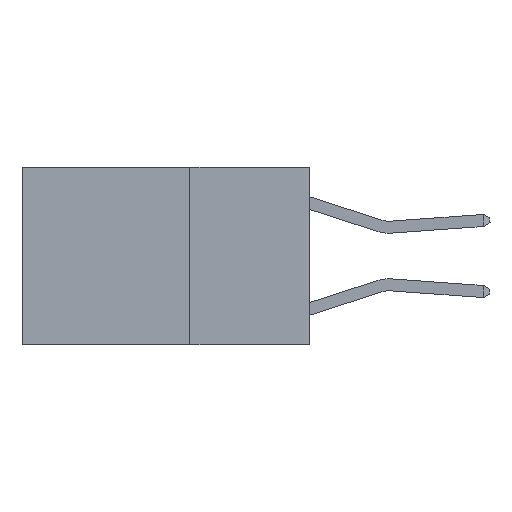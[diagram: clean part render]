
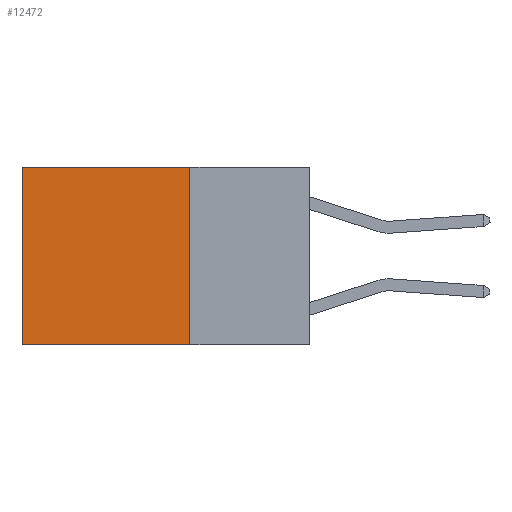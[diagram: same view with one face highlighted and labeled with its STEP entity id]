
A CAD part, left-side view. The second image highlights one B-rep face of the part: STEP entity #12472.
In plain terms, the highlighted planar face has unit normal (-1, 0, 0).
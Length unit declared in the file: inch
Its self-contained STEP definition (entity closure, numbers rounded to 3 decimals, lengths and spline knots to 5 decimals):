
#630 = CARTESIAN_POINT ( 'NONE',  ( 0.2625, 0.25, 0. ) ) ;
#1716 = LINE ( 'NONE', #6761, #12873 ) ;
#1860 = VECTOR ( 'NONE', #16292, 39.37008 ) ;
#2094 = VERTEX_POINT ( 'NONE', #2474 ) ;
#2474 = CARTESIAN_POINT ( 'NONE',  ( 0.2625, 0.6, -0.37 ) ) ;
#2919 = FACE_OUTER_BOUND ( 'NONE', #8704, .T. ) ;
#2928 = LINE ( 'NONE', #9169, #17981 ) ;
#3187 = CARTESIAN_POINT ( 'NONE',  ( 0.2625, 0.25, 0. ) ) ;
#3394 = ORIENTED_EDGE ( 'NONE', *, *, #8273, .F. ) ;
#3445 = CARTESIAN_POINT ( 'NONE',  ( 0.2625, 0.25, -0.37 ) ) ;
#4412 = VERTEX_POINT ( 'NONE', #630 ) ;
#4637 = DIRECTION ( 'NONE',  ( 0., 0., -1. ) ) ;
#4895 = CARTESIAN_POINT ( 'NONE',  ( 0.2625, 0.25, 0. ) ) ;
#5557 = EDGE_CURVE ( 'NONE', #10922, #2094, #6186, .T. ) ;
#6102 = ORIENTED_EDGE ( 'NONE', *, *, #14836, .F. ) ;
#6186 = LINE ( 'NONE', #14834, #1860 ) ;
#6761 = CARTESIAN_POINT ( 'NONE',  ( 0.2625, 0.25, -0.37 ) ) ;
#7015 = ORIENTED_EDGE ( 'NONE', *, *, #5557, .T. ) ;
#8207 = AXIS2_PLACEMENT_3D ( 'NONE', #3187, #13376, #4637 ) ;
#8273 = EDGE_CURVE ( 'NONE', #4412, #16654, #2928, .T. ) ;
#8330 = EDGE_CURVE ( 'NONE', #4412, #10922, #9289, .T. ) ;
#8704 = EDGE_LOOP ( 'NONE', ( #7015, #6102, #3394, #10443 ) ) ;
#8967 = PLANE ( 'NONE',  #8207 ) ;
#9169 = CARTESIAN_POINT ( 'NONE',  ( 0.2625, 0.25, 0. ) ) ;
#9231 = DIRECTION ( 'NONE',  ( 0., 1., 0. ) ) ;
#9289 = LINE ( 'NONE', #4895, #17505 ) ;
#10443 = ORIENTED_EDGE ( 'NONE', *, *, #8330, .T. ) ;
#10922 = VERTEX_POINT ( 'NONE', #15137 ) ;
#11141 = DIRECTION ( 'NONE',  ( 0., 1., 0. ) ) ;
#12042 = DIRECTION ( 'NONE',  ( 0., 0., -1. ) ) ;
#12472 = ADVANCED_FACE ( 'NONE', ( #2919 ), #8967, .F. ) ;
#12873 = VECTOR ( 'NONE', #11141, 39.37008 ) ;
#13376 = DIRECTION ( 'NONE',  ( 1., 0., 0. ) ) ;
#14834 = CARTESIAN_POINT ( 'NONE',  ( 0.2625, 0.6, 0. ) ) ;
#14836 = EDGE_CURVE ( 'NONE', #16654, #2094, #1716, .T. ) ;
#15137 = CARTESIAN_POINT ( 'NONE',  ( 0.2625, 0.6, 0. ) ) ;
#16292 = DIRECTION ( 'NONE',  ( 0., 0., -1. ) ) ;
#16654 = VERTEX_POINT ( 'NONE', #3445 ) ;
#17505 = VECTOR ( 'NONE', #9231, 39.37008 ) ;
#17981 = VECTOR ( 'NONE', #12042, 39.37008 ) ;
